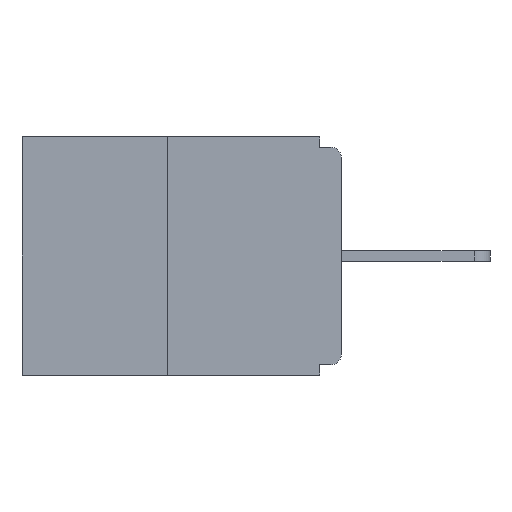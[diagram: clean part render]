
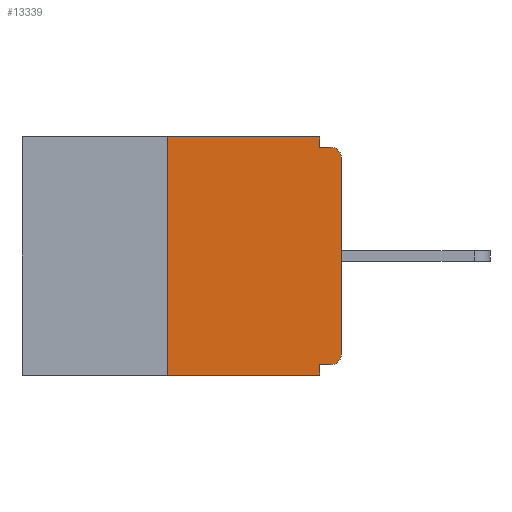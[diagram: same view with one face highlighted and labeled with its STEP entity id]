
A CAD part, left-side view. The second image highlights one B-rep face of the part: STEP entity #13339.
In plain terms, the highlighted planar face has unit normal (-1, 0, 0).
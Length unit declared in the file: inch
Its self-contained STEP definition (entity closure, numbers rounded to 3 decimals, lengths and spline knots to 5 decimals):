
#49 = VERTEX_POINT ( 'NONE', #12691 ) ;
#347 = CARTESIAN_POINT ( 'NONE',  ( 0., 0.031, -0.343 ) ) ;
#452 = DIRECTION ( 'NONE',  ( 0., 0., -1. ) ) ;
#874 = ORIENTED_EDGE ( 'NONE', *, *, #10590, .F. ) ;
#1264 = LINE ( 'NONE', #7131, #7353 ) ;
#1301 = CARTESIAN_POINT ( 'NONE',  ( 0., 0.031, 0. ) ) ;
#1425 = EDGE_CURVE ( 'NONE', #7736, #10774, #6670, .T. ) ;
#1681 = DIRECTION ( 'NONE',  ( 0., 0., -1. ) ) ;
#1824 = LINE ( 'NONE', #347, #10782 ) ;
#1850 = CARTESIAN_POINT ( 'NONE',  ( 0., 0.25, -0.343 ) ) ;
#2202 = VERTEX_POINT ( 'NONE', #1850 ) ;
#2282 = VECTOR ( 'NONE', #4518, 39.37008 ) ;
#2653 = LINE ( 'NONE', #10176, #2282 ) ;
#2891 = LINE ( 'NONE', #12647, #8632 ) ;
#3031 = LINE ( 'NONE', #11384, #5626 ) ;
#3218 = ORIENTED_EDGE ( 'NONE', *, *, #11260, .F. ) ;
#3362 = VECTOR ( 'NONE', #7004, 39.37008 ) ;
#3567 = ORIENTED_EDGE ( 'NONE', *, *, #1425, .T. ) ;
#4091 = CARTESIAN_POINT ( 'NONE',  ( 0., 0.031, -0.343 ) ) ;
#4437 = LINE ( 'NONE', #5807, #3362 ) ;
#4518 = DIRECTION ( 'NONE',  ( 0., 0., 1. ) ) ;
#4618 = DIRECTION ( 'NONE',  ( 1., 0., 0. ) ) ;
#4749 = EDGE_CURVE ( 'NONE', #10774, #49, #12397, .T. ) ;
#4954 = FACE_OUTER_BOUND ( 'NONE', #9106, .T. ) ;
#5227 = CARTESIAN_POINT ( 'NONE',  ( 0., 0.25, 0. ) ) ;
#5479 = VERTEX_POINT ( 'NONE', #5765 ) ;
#5626 = VECTOR ( 'NONE', #12363, 39.37008 ) ;
#5648 = VERTEX_POINT ( 'NONE', #7316 ) ;
#5765 = CARTESIAN_POINT ( 'NONE',  ( 0., 0.031, -0.015 ) ) ;
#5807 = CARTESIAN_POINT ( 'NONE',  ( 0., 0., -0.015 ) ) ;
#5828 = ORIENTED_EDGE ( 'NONE', *, *, #10456, .F. ) ;
#5954 = AXIS2_PLACEMENT_3D ( 'NONE', #11408, #11448, #13563 ) ;
#6066 = AXIS2_PLACEMENT_3D ( 'NONE', #13599, #7310, #452 ) ;
#6195 = ORIENTED_EDGE ( 'NONE', *, *, #11440, .F. ) ;
#6222 = CARTESIAN_POINT ( 'NONE',  ( 0., 0., -0.328 ) ) ;
#6242 = EDGE_CURVE ( 'NONE', #5648, #7736, #13416, .T. ) ;
#6670 = LINE ( 'NONE', #11993, #14083 ) ;
#6917 = VERTEX_POINT ( 'NONE', #4091 ) ;
#7004 = DIRECTION ( 'NONE',  ( 0., -1., 0. ) ) ;
#7131 = CARTESIAN_POINT ( 'NONE',  ( 0., 0.46, 0. ) ) ;
#7216 = DIRECTION ( 'NONE',  ( 0., 0., -1. ) ) ;
#7310 = DIRECTION ( 'NONE',  ( -1., 0., 0. ) ) ;
#7316 = CARTESIAN_POINT ( 'NONE',  ( 0., 0.015, -0.328 ) ) ;
#7353 = VECTOR ( 'NONE', #13453, 39.37008 ) ;
#7736 = VERTEX_POINT ( 'NONE', #7897 ) ;
#7851 = EDGE_CURVE ( 'NONE', #5479, #49, #4437, .T. ) ;
#7897 = CARTESIAN_POINT ( 'NONE',  ( 0., 0., -0.313 ) ) ;
#8580 = VERTEX_POINT ( 'NONE', #1301 ) ;
#8632 = VECTOR ( 'NONE', #1681, 39.37008 ) ;
#8952 = ORIENTED_EDGE ( 'NONE', *, *, #13263, .F. ) ;
#9106 = EDGE_LOOP ( 'NONE', ( #5828, #8952, #11730, #3218, #6195, #12049, #3567, #9614, #12354, #874 ) ) ;
#9464 = LINE ( 'NONE', #6222, #14154 ) ;
#9614 = ORIENTED_EDGE ( 'NONE', *, *, #4749, .T. ) ;
#9988 = VERTEX_POINT ( 'NONE', #5227 ) ;
#10176 = CARTESIAN_POINT ( 'NONE',  ( 0., 0.25, 0. ) ) ;
#10456 = EDGE_CURVE ( 'NONE', #9988, #8580, #1264, .T. ) ;
#10590 = EDGE_CURVE ( 'NONE', #8580, #5479, #2891, .T. ) ;
#10774 = VERTEX_POINT ( 'NONE', #10850 ) ;
#10782 = VECTOR ( 'NONE', #7216, 39.37008 ) ;
#10850 = CARTESIAN_POINT ( 'NONE',  ( 0., 0., -0.03 ) ) ;
#11068 = VERTEX_POINT ( 'NONE', #14233 ) ;
#11260 = EDGE_CURVE ( 'NONE', #11068, #6917, #1824, .T. ) ;
#11279 = PLANE ( 'NONE',  #13977 ) ;
#11384 = CARTESIAN_POINT ( 'NONE',  ( 0., 0.46, -0.343 ) ) ;
#11408 = CARTESIAN_POINT ( 'NONE',  ( 0., 0.015, -0.03 ) ) ;
#11440 = EDGE_CURVE ( 'NONE', #5648, #11068, #9464, .T. ) ;
#11448 = DIRECTION ( 'NONE',  ( -1., 0., 0. ) ) ;
#11709 = DIRECTION ( 'NONE',  ( 0., 0., 1. ) ) ;
#11730 = ORIENTED_EDGE ( 'NONE', *, *, #12608, .T. ) ;
#11993 = CARTESIAN_POINT ( 'NONE',  ( 0., 0., 0. ) ) ;
#12049 = ORIENTED_EDGE ( 'NONE', *, *, #6242, .T. ) ;
#12305 = DIRECTION ( 'NONE',  ( 0., 0., -1. ) ) ;
#12354 = ORIENTED_EDGE ( 'NONE', *, *, #7851, .F. ) ;
#12363 = DIRECTION ( 'NONE',  ( 0., -1., 0. ) ) ;
#12397 = CIRCLE ( 'NONE', #5954, 0.015 ) ;
#12608 = EDGE_CURVE ( 'NONE', #2202, #6917, #3031, .T. ) ;
#12647 = CARTESIAN_POINT ( 'NONE',  ( 0., 0.031, 0. ) ) ;
#12691 = CARTESIAN_POINT ( 'NONE',  ( 0., 0.015, -0.015 ) ) ;
#12767 = DIRECTION ( 'NONE',  ( 0., 1., 0. ) ) ;
#13237 = CARTESIAN_POINT ( 'NONE',  ( 0., 0.46, 0. ) ) ;
#13263 = EDGE_CURVE ( 'NONE', #2202, #9988, #2653, .T. ) ;
#13339 = ADVANCED_FACE ( 'NONE', ( #4954 ), #11279, .F. ) ;
#13416 = CIRCLE ( 'NONE', #6066, 0.015 ) ;
#13453 = DIRECTION ( 'NONE',  ( 0., -1., 0. ) ) ;
#13563 = DIRECTION ( 'NONE',  ( 0., 0., -1. ) ) ;
#13599 = CARTESIAN_POINT ( 'NONE',  ( 0., 0.015, -0.313 ) ) ;
#13977 = AXIS2_PLACEMENT_3D ( 'NONE', #13237, #4618, #12305 ) ;
#14083 = VECTOR ( 'NONE', #11709, 39.37008 ) ;
#14154 = VECTOR ( 'NONE', #12767, 39.37008 ) ;
#14233 = CARTESIAN_POINT ( 'NONE',  ( 0., 0.031, -0.328 ) ) ;
